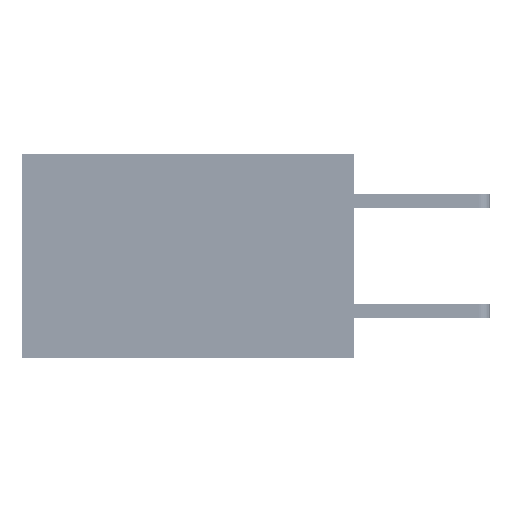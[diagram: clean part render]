
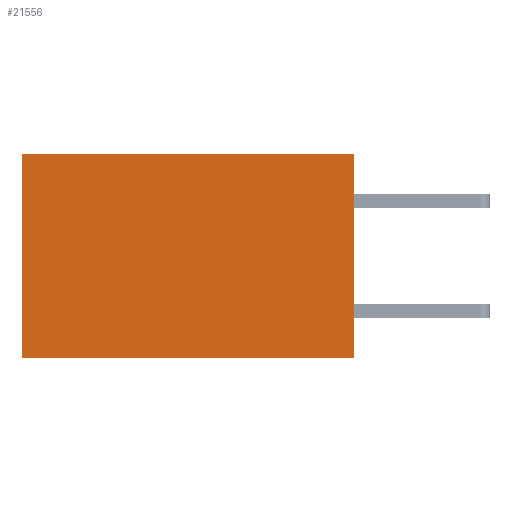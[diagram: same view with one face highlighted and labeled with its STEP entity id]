
A CAD part, left-side view. The second image highlights one B-rep face of the part: STEP entity #21556.
In plain terms, the highlighted planar face has unit normal (-1, 0, 0).
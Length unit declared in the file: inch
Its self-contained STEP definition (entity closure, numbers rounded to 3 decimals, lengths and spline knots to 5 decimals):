
#444 = CARTESIAN_POINT ( 'NONE',  ( 0.2875, 0., 0. ) ) ;
#1175 = DIRECTION ( 'NONE',  ( 0., 1., 0. ) ) ;
#1564 = VERTEX_POINT ( 'NONE', #14482 ) ;
#2204 = EDGE_CURVE ( 'NONE', #23416, #23427, #36898, .T. ) ;
#2433 = VECTOR ( 'NONE', #1175, 39.37008 ) ;
#2484 = EDGE_CURVE ( 'NONE', #1564, #21867, #30852, .T. ) ;
#2628 = DIRECTION ( 'NONE',  ( 0., 1., 0. ) ) ;
#4391 = ORIENTED_EDGE ( 'NONE', *, *, #17967, .F. ) ;
#5468 = ORIENTED_EDGE ( 'NONE', *, *, #20941, .T. ) ;
#5683 = DIRECTION ( 'NONE',  ( 0., 0., -1. ) ) ;
#12148 = CARTESIAN_POINT ( 'NONE',  ( 0.2875, 0.6, 0. ) ) ;
#12277 = VECTOR ( 'NONE', #2628, 39.37008 ) ;
#14482 = CARTESIAN_POINT ( 'NONE',  ( 0.2875, 0., -0.37 ) ) ;
#15038 = DIRECTION ( 'NONE',  ( 0., 0., -1. ) ) ;
#15072 = ORIENTED_EDGE ( 'NONE', *, *, #2204, .T. ) ;
#16416 = VECTOR ( 'NONE', #5683, 39.37008 ) ;
#17813 = CARTESIAN_POINT ( 'NONE',  ( 0.2875, 0., 0. ) ) ;
#17967 = EDGE_CURVE ( 'NONE', #23416, #1564, #24816, .T. ) ;
#18086 = CARTESIAN_POINT ( 'NONE',  ( 0.2875, 0.6, 0. ) ) ;
#20237 = PLANE ( 'NONE',  #27948 ) ;
#20603 = DIRECTION ( 'NONE',  ( 1., 0., 0. ) ) ;
#20823 = ORIENTED_EDGE ( 'NONE', *, *, #2484, .F. ) ;
#20941 = EDGE_CURVE ( 'NONE', #23427, #21867, #22285, .T. ) ;
#21556 = ADVANCED_FACE ( 'NONE', ( #29267 ), #20237, .F. ) ;
#21867 = VERTEX_POINT ( 'NONE', #30230 ) ;
#22285 = LINE ( 'NONE', #18086, #36723 ) ;
#23416 = VERTEX_POINT ( 'NONE', #444 ) ;
#23427 = VERTEX_POINT ( 'NONE', #12148 ) ;
#24816 = LINE ( 'NONE', #17813, #16416 ) ;
#24837 = CARTESIAN_POINT ( 'NONE',  ( 0.2875, 0., -0.37 ) ) ;
#26202 = CARTESIAN_POINT ( 'NONE',  ( 0.2875, 0., 0. ) ) ;
#27948 = AXIS2_PLACEMENT_3D ( 'NONE', #26202, #20603, #38241 ) ;
#29267 = FACE_OUTER_BOUND ( 'NONE', #38416, .T. ) ;
#30230 = CARTESIAN_POINT ( 'NONE',  ( 0.2875, 0.6, -0.37 ) ) ;
#30852 = LINE ( 'NONE', #24837, #2433 ) ;
#35500 = CARTESIAN_POINT ( 'NONE',  ( 0.2875, 0., 0. ) ) ;
#36723 = VECTOR ( 'NONE', #15038, 39.37008 ) ;
#36898 = LINE ( 'NONE', #35500, #12277 ) ;
#38241 = DIRECTION ( 'NONE',  ( 0., 0., -1. ) ) ;
#38416 = EDGE_LOOP ( 'NONE', ( #5468, #20823, #4391, #15072 ) ) ;
